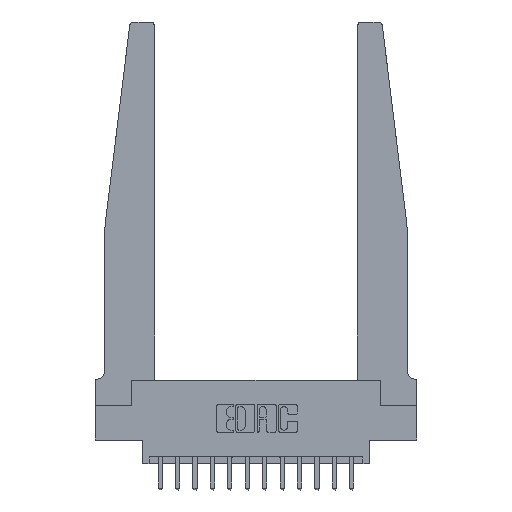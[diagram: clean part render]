
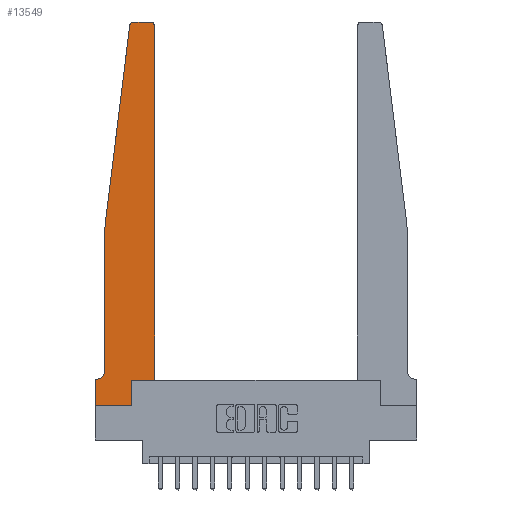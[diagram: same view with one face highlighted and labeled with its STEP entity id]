
A CAD part, top view. The second image highlights one B-rep face of the part: STEP entity #13549.
In plain terms, the highlighted planar face has unit normal (0, 0, 1).
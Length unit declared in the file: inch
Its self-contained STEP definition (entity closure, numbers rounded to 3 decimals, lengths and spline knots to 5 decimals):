
#43 = CARTESIAN_POINT ( 'NONE',  ( 0.425, 0.18, 0.37 ) ) ;
#53 = LINE ( 'NONE', #12085, #10631 ) ;
#420 = DIRECTION ( 'NONE',  ( 1., 0., 0. ) ) ;
#565 = EDGE_CURVE ( 'NONE', #6707, #4645, #13772, .T. ) ;
#1166 = LINE ( 'NONE', #6548, #10283 ) ;
#1925 = CARTESIAN_POINT ( 'NONE',  ( 0.425, 2.72, 0.37 ) ) ;
#1991 = ORIENTED_EDGE ( 'NONE', *, *, #17294, .T. ) ;
#2089 = DIRECTION ( 'NONE',  ( 1., 0., 0. ) ) ;
#2256 = EDGE_CURVE ( 'NONE', #14683, #7660, #11716, .T. ) ;
#2257 = VECTOR ( 'NONE', #13773, 39.37008 ) ;
#2334 = VECTOR ( 'NONE', #11044, 39.37008 ) ;
#2916 = DIRECTION ( 'NONE',  ( 0., 0., -1. ) ) ;
#3185 = DIRECTION ( 'NONE',  ( -1., 0., 0. ) ) ;
#3258 = CARTESIAN_POINT ( 'NONE',  ( 0.395, 2.75, 0.37 ) ) ;
#3278 = EDGE_CURVE ( 'NONE', #12798, #12630, #6216, .T. ) ;
#3292 = ORIENTED_EDGE ( 'NONE', *, *, #13133, .T. ) ;
#3654 = VECTOR ( 'NONE', #15238, 39.37008 ) ;
#3830 = CARTESIAN_POINT ( 'NONE',  ( 0.065, 0.1875, 0.37 ) ) ;
#3869 = AXIS2_PLACEMENT_3D ( 'NONE', #13977, #8800, #2089 ) ;
#3889 = CARTESIAN_POINT ( 'NONE',  ( 0.24675, 2.72367, 0.37 ) ) ;
#4176 = DIRECTION ( 'NONE',  ( 1., 0., 0. ) ) ;
#4277 = CARTESIAN_POINT ( 'NONE',  ( 0.065, 1.25, 0.37 ) ) ;
#4461 = CARTESIAN_POINT ( 'NONE',  ( 0.425, 0.18, 0.37 ) ) ;
#4645 = VERTEX_POINT ( 'NONE', #7982 ) ;
#4656 = VERTEX_POINT ( 'NONE', #12091 ) ;
#4706 = CARTESIAN_POINT ( 'NONE',  ( 0.015, 0.1875, 0.37 ) ) ;
#4724 = CARTESIAN_POINT ( 'NONE',  ( 0.2605, 0., 0.37 ) ) ;
#4767 = EDGE_CURVE ( 'NONE', #9679, #16387, #5781, .T. ) ;
#4825 = VERTEX_POINT ( 'NONE', #12786 ) ;
#5163 = VECTOR ( 'NONE', #4176, 39.37008 ) ;
#5781 = LINE ( 'NONE', #4461, #2334 ) ;
#5843 = AXIS2_PLACEMENT_3D ( 'NONE', #15210, #2916, #3185 ) ;
#5970 = DIRECTION ( 'NONE',  ( 1., 0., 0. ) ) ;
#6216 = LINE ( 'NONE', #3830, #14685 ) ;
#6273 = EDGE_CURVE ( 'NONE', #4825, #9679, #15836, .T. ) ;
#6394 = CIRCLE ( 'NONE', #5843, 0.05 ) ;
#6471 = DIRECTION ( 'NONE',  ( -1., 0., 0. ) ) ;
#6548 = CARTESIAN_POINT ( 'NONE',  ( 0.065, 1.25, 0.37 ) ) ;
#6707 = VERTEX_POINT ( 'NONE', #3889 ) ;
#6865 = ORIENTED_EDGE ( 'NONE', *, *, #4767, .T. ) ;
#7302 = ORIENTED_EDGE ( 'NONE', *, *, #2256, .T. ) ;
#7401 = FACE_OUTER_BOUND ( 'NONE', #16127, .T. ) ;
#7466 = ORIENTED_EDGE ( 'NONE', *, *, #9222, .T. ) ;
#7660 = VERTEX_POINT ( 'NONE', #4724 ) ;
#7735 = ORIENTED_EDGE ( 'NONE', *, *, #14248, .T. ) ;
#7957 = CARTESIAN_POINT ( 'NONE',  ( 0.425, 0.18, 0.37 ) ) ;
#7975 = DIRECTION ( 'NONE',  ( 0., -1., 0. ) ) ;
#7982 = CARTESIAN_POINT ( 'NONE',  ( 0.065, 1.25, 0.37 ) ) ;
#8116 = CARTESIAN_POINT ( 'NONE',  ( 0.27653, 2.72, 0.37 ) ) ;
#8525 = DIRECTION ( 'NONE',  ( 0., 0., 1. ) ) ;
#8541 = ORIENTED_EDGE ( 'NONE', *, *, #10093, .T. ) ;
#8633 = CIRCLE ( 'NONE', #13652, 0.03 ) ;
#8800 = DIRECTION ( 'NONE',  ( 0., 0., 1. ) ) ;
#8840 = CARTESIAN_POINT ( 'NONE',  ( 0., 0., 0.37 ) ) ;
#9009 = EDGE_CURVE ( 'NONE', #16387, #16450, #12783, .T. ) ;
#9180 = ORIENTED_EDGE ( 'NONE', *, *, #3278, .T. ) ;
#9222 = EDGE_CURVE ( 'NONE', #4645, #4656, #1166, .T. ) ;
#9679 = VERTEX_POINT ( 'NONE', #7957 ) ;
#10021 = DIRECTION ( 'NONE',  ( 0., 0., 1. ) ) ;
#10093 = EDGE_CURVE ( 'NONE', #15773, #6707, #8633, .T. ) ;
#10233 = CARTESIAN_POINT ( 'NONE',  ( 0.25, 2.75, 0.37 ) ) ;
#10283 = VECTOR ( 'NONE', #7975, 39.37008 ) ;
#10481 = CARTESIAN_POINT ( 'NONE',  ( 0., 0., 0.37 ) ) ;
#10631 = VECTOR ( 'NONE', #10778, 39.37008 ) ;
#10778 = DIRECTION ( 'NONE',  ( 0., -1., 0. ) ) ;
#11044 = DIRECTION ( 'NONE',  ( 0., 1., 0. ) ) ;
#11261 = VECTOR ( 'NONE', #17033, 39.37008 ) ;
#11613 = DIRECTION ( 'NONE',  ( 0., 1., 0. ) ) ;
#11654 = ORIENTED_EDGE ( 'NONE', *, *, #565, .T. ) ;
#11716 = LINE ( 'NONE', #8840, #11261 ) ;
#11805 = VECTOR ( 'NONE', #11613, 39.37008 ) ;
#11883 = LINE ( 'NONE', #17197, #11805 ) ;
#12085 = CARTESIAN_POINT ( 'NONE',  ( 0., 0., 0.37 ) ) ;
#12091 = CARTESIAN_POINT ( 'NONE',  ( 0.065, 0.2375, 0.37 ) ) ;
#12630 = VERTEX_POINT ( 'NONE', #15057 ) ;
#12783 = CIRCLE ( 'NONE', #15014, 0.03 ) ;
#12786 = CARTESIAN_POINT ( 'NONE',  ( 0.2605, 0.18, 0.37 ) ) ;
#12798 = VERTEX_POINT ( 'NONE', #4706 ) ;
#12865 = ORIENTED_EDGE ( 'NONE', *, *, #16148, .T. ) ;
#13133 = EDGE_CURVE ( 'NONE', #4656, #12798, #6394, .T. ) ;
#13549 = ADVANCED_FACE ( 'NONE', ( #7401 ), #15355, .T. ) ;
#13652 = AXIS2_PLACEMENT_3D ( 'NONE', #8116, #8525, #420 ) ;
#13772 = LINE ( 'NONE', #4277, #3654 ) ;
#13773 = DIRECTION ( 'NONE',  ( -1., 0., 0. ) ) ;
#13977 = CARTESIAN_POINT ( 'NONE',  ( 0., 0.1875, 0.37 ) ) ;
#14248 = EDGE_CURVE ( 'NONE', #12630, #14683, #53, .T. ) ;
#14260 = LINE ( 'NONE', #10233, #2257 ) ;
#14683 = VERTEX_POINT ( 'NONE', #10481 ) ;
#14685 = VECTOR ( 'NONE', #6471, 39.37008 ) ;
#14927 = ORIENTED_EDGE ( 'NONE', *, *, #6273, .T. ) ;
#15014 = AXIS2_PLACEMENT_3D ( 'NONE', #16717, #10021, #5970 ) ;
#15057 = CARTESIAN_POINT ( 'NONE',  ( 0., 0.1875, 0.37 ) ) ;
#15210 = CARTESIAN_POINT ( 'NONE',  ( 0.015, 0.2375, 0.37 ) ) ;
#15235 = CARTESIAN_POINT ( 'NONE',  ( 0.27653, 2.75, 0.37 ) ) ;
#15238 = DIRECTION ( 'NONE',  ( -0.122, -0.992, 0. ) ) ;
#15355 = PLANE ( 'NONE',  #3869 ) ;
#15773 = VERTEX_POINT ( 'NONE', #15235 ) ;
#15836 = LINE ( 'NONE', #43, #5163 ) ;
#16127 = EDGE_LOOP ( 'NONE', ( #1991, #8541, #11654, #7466, #3292, #9180, #7735, #7302, #12865, #14927, #6865, #16523 ) ) ;
#16148 = EDGE_CURVE ( 'NONE', #7660, #4825, #11883, .T. ) ;
#16387 = VERTEX_POINT ( 'NONE', #1925 ) ;
#16450 = VERTEX_POINT ( 'NONE', #3258 ) ;
#16523 = ORIENTED_EDGE ( 'NONE', *, *, #9009, .T. ) ;
#16717 = CARTESIAN_POINT ( 'NONE',  ( 0.395, 2.72, 0.37 ) ) ;
#17033 = DIRECTION ( 'NONE',  ( 1., 0., 0. ) ) ;
#17197 = CARTESIAN_POINT ( 'NONE',  ( 0.2605, 0.18, 0.37 ) ) ;
#17294 = EDGE_CURVE ( 'NONE', #16450, #15773, #14260, .T. ) ;
